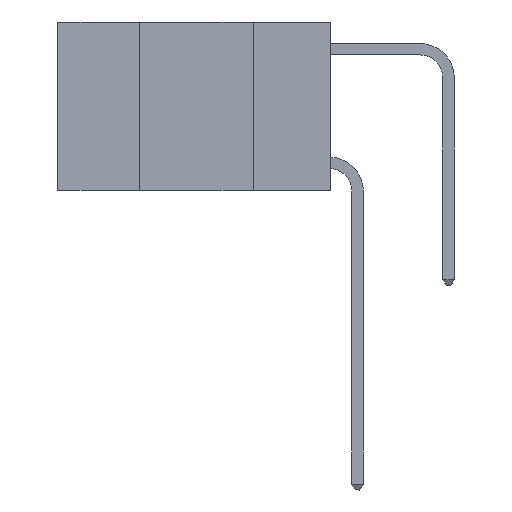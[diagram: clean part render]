
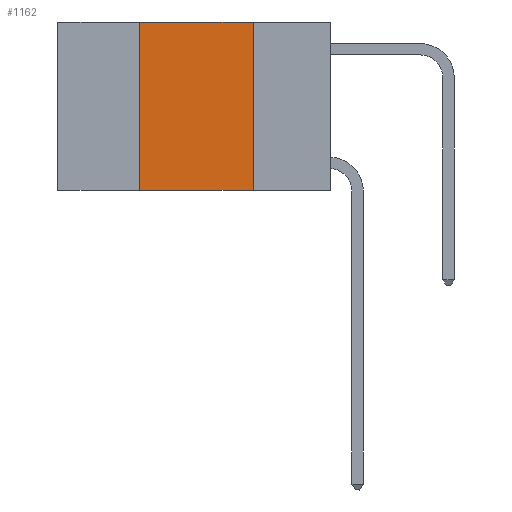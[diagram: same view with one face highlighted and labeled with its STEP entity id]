
A CAD part, left-side view. The second image highlights one B-rep face of the part: STEP entity #1162.
In plain terms, the highlighted planar face has unit normal (-1, 0, 0).
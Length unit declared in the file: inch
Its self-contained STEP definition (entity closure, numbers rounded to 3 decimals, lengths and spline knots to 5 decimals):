
#806 = LINE ( 'NONE', #2560, #20436 ) ;
#1131 = CARTESIAN_POINT ( 'NONE',  ( 0., 0.42, 0. ) ) ;
#1162 = ADVANCED_FACE ( 'NONE', ( #7306 ), #15578, .F. ) ;
#2069 = LINE ( 'NONE', #2390, #11931 ) ;
#2390 = CARTESIAN_POINT ( 'NONE',  ( 0., 0.6, 0. ) ) ;
#2560 = CARTESIAN_POINT ( 'NONE',  ( 0., 0.17, 0. ) ) ;
#3836 = CARTESIAN_POINT ( 'NONE',  ( 0., 0.6, 0. ) ) ;
#4069 = VECTOR ( 'NONE', #16181, 39.37008 ) ;
#4378 = VECTOR ( 'NONE', #9092, 39.37008 ) ;
#4461 = CARTESIAN_POINT ( 'NONE',  ( 0., 0.6, -0.37 ) ) ;
#4546 = DIRECTION ( 'NONE',  ( 0., 0., -1. ) ) ;
#5854 = DIRECTION ( 'NONE',  ( 1., 0., 0. ) ) ;
#6987 = VERTEX_POINT ( 'NONE', #15680 ) ;
#7306 = FACE_OUTER_BOUND ( 'NONE', #24629, .T. ) ;
#8202 = EDGE_CURVE ( 'NONE', #12990, #17267, #19689, .T. ) ;
#8436 = EDGE_CURVE ( 'NONE', #12990, #13495, #8985, .T. ) ;
#8985 = LINE ( 'NONE', #20756, #4378 ) ;
#9092 = DIRECTION ( 'NONE',  ( 0., 0., 1. ) ) ;
#10552 = CARTESIAN_POINT ( 'NONE',  ( 0., 0.42, -0.37 ) ) ;
#11002 = EDGE_CURVE ( 'NONE', #13495, #6987, #2069, .T. ) ;
#11049 = EDGE_CURVE ( 'NONE', #6987, #17267, #806, .T. ) ;
#11931 = VECTOR ( 'NONE', #14146, 39.37008 ) ;
#12990 = VERTEX_POINT ( 'NONE', #10552 ) ;
#13495 = VERTEX_POINT ( 'NONE', #1131 ) ;
#14146 = DIRECTION ( 'NONE',  ( 0., -1., 0. ) ) ;
#15065 = AXIS2_PLACEMENT_3D ( 'NONE', #3836, #5854, #19504 ) ;
#15578 = PLANE ( 'NONE',  #15065 ) ;
#15680 = CARTESIAN_POINT ( 'NONE',  ( 0., 0.17, 0. ) ) ;
#16181 = DIRECTION ( 'NONE',  ( 0., -1., 0. ) ) ;
#16565 = ORIENTED_EDGE ( 'NONE', *, *, #11049, .F. ) ;
#16657 = ORIENTED_EDGE ( 'NONE', *, *, #11002, .F. ) ;
#17153 = ORIENTED_EDGE ( 'NONE', *, *, #8436, .F. ) ;
#17180 = ORIENTED_EDGE ( 'NONE', *, *, #8202, .T. ) ;
#17267 = VERTEX_POINT ( 'NONE', #22011 ) ;
#19504 = DIRECTION ( 'NONE',  ( 0., 0., -1. ) ) ;
#19689 = LINE ( 'NONE', #4461, #4069 ) ;
#20436 = VECTOR ( 'NONE', #4546, 39.37008 ) ;
#20756 = CARTESIAN_POINT ( 'NONE',  ( 0., 0.42, 0. ) ) ;
#22011 = CARTESIAN_POINT ( 'NONE',  ( 0., 0.17, -0.37 ) ) ;
#24629 = EDGE_LOOP ( 'NONE', ( #16565, #16657, #17153, #17180 ) ) ;
